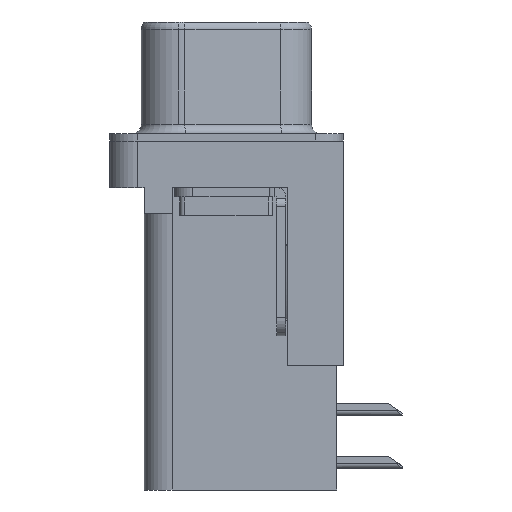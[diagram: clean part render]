
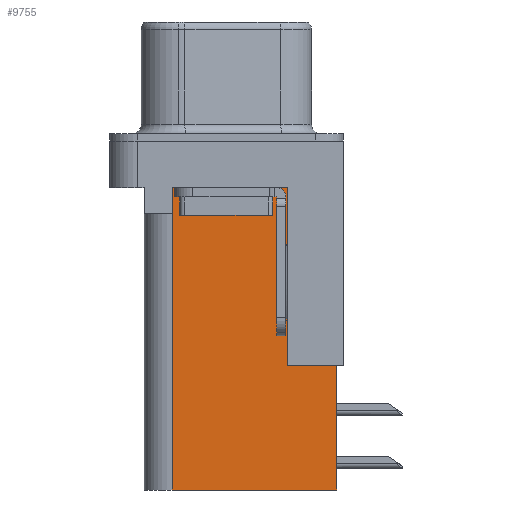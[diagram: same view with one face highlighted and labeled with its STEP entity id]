
A CAD part, left-side view. The second image highlights one B-rep face of the part: STEP entity #9755.
In plain terms, the highlighted planar face has unit normal (-1, 0, 0).
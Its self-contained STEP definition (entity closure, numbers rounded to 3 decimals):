
#613 = VERTEX_POINT ( 'NONE', #8627 ) ;
#717 = EDGE_CURVE ( 'NONE', #10576, #13619, #6407, .T. ) ;
#844 = ORIENTED_EDGE ( 'NONE', *, *, #14375, .F. ) ;
#1132 = CARTESIAN_POINT ( 'NONE',  ( 3.79, -3.295, -12.05 ) ) ;
#1150 = LINE ( 'NONE', #15061, #13783 ) ;
#1184 = PLANE ( 'NONE',  #12266 ) ;
#1446 = DIRECTION ( 'NONE',  ( 0., 1., 0. ) ) ;
#1551 = CARTESIAN_POINT ( 'NONE',  ( 3.79, -3.295, -18.76 ) ) ;
#1582 = VERTEX_POINT ( 'NONE', #7715 ) ;
#2248 = EDGE_CURVE ( 'NONE', #10576, #613, #13421, .T. ) ;
#2358 = DIRECTION ( 'NONE',  ( 0., 1., 0. ) ) ;
#2373 = ORIENTED_EDGE ( 'NONE', *, *, #13280, .T. ) ;
#2492 = CARTESIAN_POINT ( 'NONE',  ( 3.79, -3.295, -2.5 ) ) ;
#2710 = VECTOR ( 'NONE', #12786, 1000. ) ;
#2802 = EDGE_CURVE ( 'NONE', #7255, #5677, #10908, .T. ) ;
#2814 = VECTOR ( 'NONE', #4063, 1000. ) ;
#3248 = VECTOR ( 'NONE', #6195, 1000. ) ;
#3534 = LINE ( 'NONE', #4319, #2710 ) ;
#3544 = VERTEX_POINT ( 'NONE', #10856 ) ;
#3653 = VECTOR ( 'NONE', #4721, 1000. ) ;
#4063 = DIRECTION ( 'NONE',  ( 0., 1., 0. ) ) ;
#4298 = DIRECTION ( 'NONE',  ( 0., 1., 0. ) ) ;
#4319 = CARTESIAN_POINT ( 'NONE',  ( 3.79, -3.295, -18.76 ) ) ;
#4444 = VECTOR ( 'NONE', #4298, 1000. ) ;
#4721 = DIRECTION ( 'NONE',  ( 0., 0., -1. ) ) ;
#5059 = CARTESIAN_POINT ( 'NONE',  ( 3.79, -5.925, -2. ) ) ;
#5639 = EDGE_LOOP ( 'NONE', ( #6943, #7324, #15779, #844, #5681, #6839, #9763, #2373 ) ) ;
#5677 = VERTEX_POINT ( 'NONE', #13399 ) ;
#5681 = ORIENTED_EDGE ( 'NONE', *, *, #8842, .F. ) ;
#6011 = DIRECTION ( 'NONE',  ( 0., 0., 1. ) ) ;
#6195 = DIRECTION ( 'NONE',  ( 0., 0., -1. ) ) ;
#6407 = LINE ( 'NONE', #10235, #15569 ) ;
#6542 = LINE ( 'NONE', #12254, #3248 ) ;
#6839 = ORIENTED_EDGE ( 'NONE', *, *, #2248, .F. ) ;
#6943 = ORIENTED_EDGE ( 'NONE', *, *, #8790, .T. ) ;
#7255 = VERTEX_POINT ( 'NONE', #7981 ) ;
#7324 = ORIENTED_EDGE ( 'NONE', *, *, #8301, .T. ) ;
#7546 = CARTESIAN_POINT ( 'NONE',  ( 3.79, 0., -3.9 ) ) ;
#7715 = CARTESIAN_POINT ( 'NONE',  ( 3.79, 2.895, -2.5 ) ) ;
#7981 = CARTESIAN_POINT ( 'NONE',  ( 3.79, 2.895, -3.9 ) ) ;
#8010 = LINE ( 'NONE', #8456, #8394 ) ;
#8301 = EDGE_CURVE ( 'NONE', #1582, #7255, #6542, .T. ) ;
#8394 = VECTOR ( 'NONE', #6011, 1000. ) ;
#8456 = CARTESIAN_POINT ( 'NONE',  ( 3.79, 2.925, -18.76 ) ) ;
#8627 = CARTESIAN_POINT ( 'NONE',  ( 3.79, -5.925, -18.76 ) ) ;
#8790 = EDGE_CURVE ( 'NONE', #15134, #1582, #1150, .T. ) ;
#8842 = EDGE_CURVE ( 'NONE', #613, #3544, #9361, .T. ) ;
#9361 = LINE ( 'NONE', #1551, #2814 ) ;
#9669 = CARTESIAN_POINT ( 'NONE',  ( 3.79, -3.295, -18.76 ) ) ;
#9713 = DIRECTION ( 'NONE',  ( 1., 0., 0. ) ) ;
#9755 = ADVANCED_FACE ( 'NONE', ( #10078 ), #1184, .F. ) ;
#9763 = ORIENTED_EDGE ( 'NONE', *, *, #717, .T. ) ;
#10078 = FACE_OUTER_BOUND ( 'NONE', #5639, .T. ) ;
#10132 = DIRECTION ( 'NONE',  ( 0., 1., 0. ) ) ;
#10235 = CARTESIAN_POINT ( 'NONE',  ( 3.79, -6.295, -12.05 ) ) ;
#10576 = VERTEX_POINT ( 'NONE', #12439 ) ;
#10856 = CARTESIAN_POINT ( 'NONE',  ( 3.79, 2.925, -18.76 ) ) ;
#10908 = LINE ( 'NONE', #7546, #4444 ) ;
#12254 = CARTESIAN_POINT ( 'NONE',  ( 3.79, 2.895, -3.9 ) ) ;
#12266 = AXIS2_PLACEMENT_3D ( 'NONE', #9669, #9713, #2358 ) ;
#12439 = CARTESIAN_POINT ( 'NONE',  ( 3.79, -5.925, -12.05 ) ) ;
#12786 = DIRECTION ( 'NONE',  ( 0., 0., 1. ) ) ;
#13280 = EDGE_CURVE ( 'NONE', #13619, #15134, #3534, .T. ) ;
#13399 = CARTESIAN_POINT ( 'NONE',  ( 3.79, 2.925, -3.9 ) ) ;
#13421 = LINE ( 'NONE', #5059, #3653 ) ;
#13619 = VERTEX_POINT ( 'NONE', #1132 ) ;
#13783 = VECTOR ( 'NONE', #1446, 1000. ) ;
#14375 = EDGE_CURVE ( 'NONE', #3544, #5677, #8010, .T. ) ;
#15061 = CARTESIAN_POINT ( 'NONE',  ( 3.79, -3.295, -2.5 ) ) ;
#15134 = VERTEX_POINT ( 'NONE', #2492 ) ;
#15569 = VECTOR ( 'NONE', #10132, 1000. ) ;
#15779 = ORIENTED_EDGE ( 'NONE', *, *, #2802, .T. ) ;
